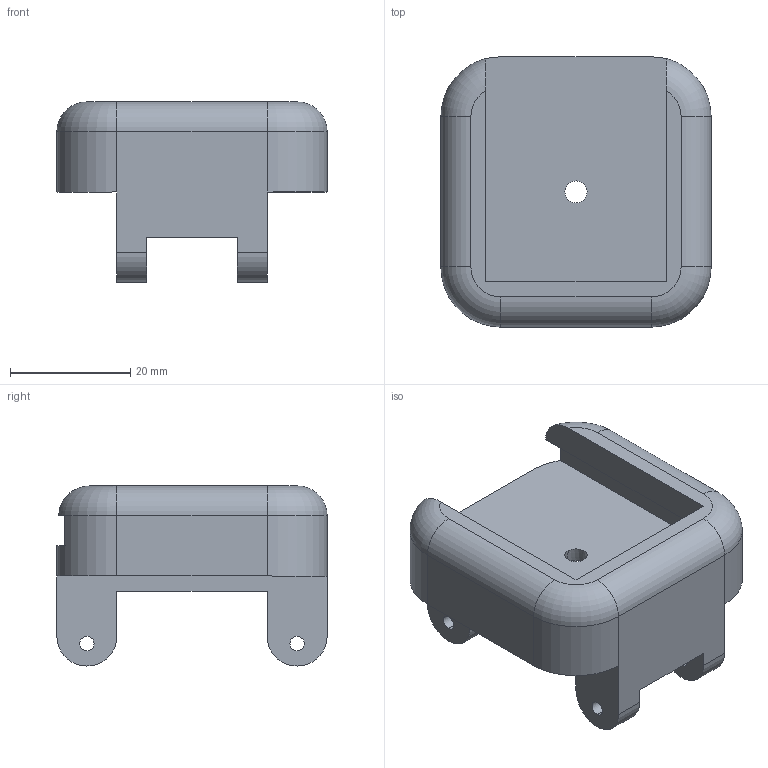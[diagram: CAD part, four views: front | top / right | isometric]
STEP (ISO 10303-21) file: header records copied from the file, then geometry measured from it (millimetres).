
FILE_DESCRIPTION (( 'STEP AP203' ), '1' );
FILE_NAME ('Hammer_Body.STEP', '2013-11-10T07:41:56', ( '' ), ( '' ), 'SwSTEP 2.0', 'SolidWorks 2013', '' );
FILE_SCHEMA (( 'CONFIG_CONTROL_DESIGN' ));
Length unit declared in the file: millimetre
Products named in the file (1): Hammer_Body
Bounding box: 45 x 45 x 30 mm (x, y, z)
Volume: 21553 mm3; surface area: 9157 mm2
Topology: 1 solids, 1 shells, 60 faces, 156 edges, 98 vertices
Faces by surface type: plane 30, cylinder 22, torus 6, cone 2
Entity records: 1967 total; most frequent: CARTESIAN_POINT 349, DIRECTION 340, ORIENTED_EDGE 312, EDGE_CURVE 156, AXIS2_PLACEMENT_3D 125, VERTEX_POINT 98, LINE 90, VECTOR 90
